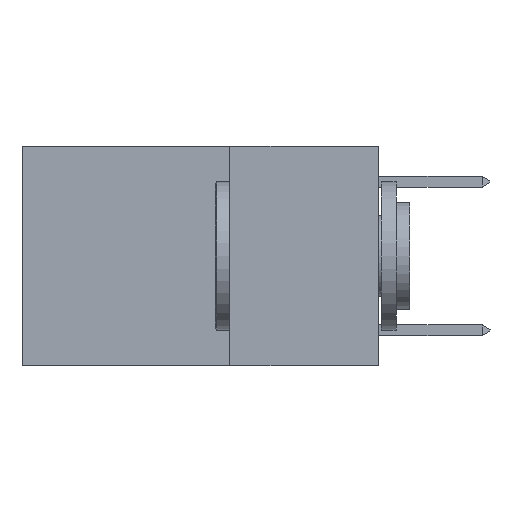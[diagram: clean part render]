
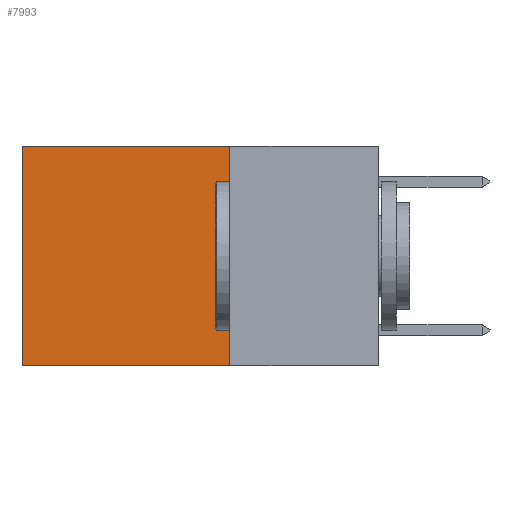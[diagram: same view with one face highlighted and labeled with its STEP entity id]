
A CAD part, left-side view. The second image highlights one B-rep face of the part: STEP entity #7993.
In plain terms, the highlighted planar face has unit normal (-1, 0, 0).
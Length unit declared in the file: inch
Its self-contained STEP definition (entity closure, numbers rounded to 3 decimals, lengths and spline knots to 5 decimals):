
#565 = CARTESIAN_POINT ( 'NONE',  ( 0.2625, 0.25, 0. ) ) ;
#1042 = DIRECTION ( 'NONE',  ( 0., 1., 0. ) ) ;
#1241 = CARTESIAN_POINT ( 'NONE',  ( 0.2625, 0.25, 0. ) ) ;
#1572 = VECTOR ( 'NONE', #13130, 39.37008 ) ;
#1951 = EDGE_CURVE ( 'NONE', #12552, #6987, #2225, .T. ) ;
#2107 = CARTESIAN_POINT ( 'NONE',  ( 0.2625, 0.6, 0. ) ) ;
#2225 = LINE ( 'NONE', #5620, #7541 ) ;
#2430 = PLANE ( 'NONE',  #9959 ) ;
#3626 = VERTEX_POINT ( 'NONE', #565 ) ;
#3913 = LINE ( 'NONE', #4499, #6541 ) ;
#4010 = DIRECTION ( 'NONE',  ( 0., 0., -1. ) ) ;
#4499 = CARTESIAN_POINT ( 'NONE',  ( 0.2625, 0.25, -0.37 ) ) ;
#4833 = EDGE_CURVE ( 'NONE', #3626, #13359, #7638, .T. ) ;
#5126 = CARTESIAN_POINT ( 'NONE',  ( 0.2625, 0.25, 0. ) ) ;
#5620 = CARTESIAN_POINT ( 'NONE',  ( 0.2625, 0.6, 0. ) ) ;
#5685 = ORIENTED_EDGE ( 'NONE', *, *, #6334, .F. ) ;
#5765 = CARTESIAN_POINT ( 'NONE',  ( 0.2625, 0.6, -0.37 ) ) ;
#6084 = LINE ( 'NONE', #5126, #14703 ) ;
#6334 = EDGE_CURVE ( 'NONE', #13359, #6987, #3913, .T. ) ;
#6541 = VECTOR ( 'NONE', #1042, 39.37008 ) ;
#6987 = VERTEX_POINT ( 'NONE', #5765 ) ;
#7541 = VECTOR ( 'NONE', #4010, 39.37008 ) ;
#7638 = LINE ( 'NONE', #12020, #1572 ) ;
#7993 = ADVANCED_FACE ( 'NONE', ( #12672 ), #2430, .F. ) ;
#8221 = EDGE_CURVE ( 'NONE', #3626, #12552, #6084, .T. ) ;
#9959 = AXIS2_PLACEMENT_3D ( 'NONE', #1241, #13712, #10430 ) ;
#10430 = DIRECTION ( 'NONE',  ( 0., 0., -1. ) ) ;
#11489 = ORIENTED_EDGE ( 'NONE', *, *, #4833, .F. ) ;
#11588 = EDGE_LOOP ( 'NONE', ( #12355, #5685, #11489, #13217 ) ) ;
#12020 = CARTESIAN_POINT ( 'NONE',  ( 0.2625, 0.25, 0. ) ) ;
#12355 = ORIENTED_EDGE ( 'NONE', *, *, #1951, .T. ) ;
#12552 = VERTEX_POINT ( 'NONE', #2107 ) ;
#12672 = FACE_OUTER_BOUND ( 'NONE', #11588, .T. ) ;
#13046 = DIRECTION ( 'NONE',  ( 0., 1., 0. ) ) ;
#13130 = DIRECTION ( 'NONE',  ( 0., 0., -1. ) ) ;
#13217 = ORIENTED_EDGE ( 'NONE', *, *, #8221, .T. ) ;
#13233 = CARTESIAN_POINT ( 'NONE',  ( 0.2625, 0.25, -0.37 ) ) ;
#13359 = VERTEX_POINT ( 'NONE', #13233 ) ;
#13712 = DIRECTION ( 'NONE',  ( 1., 0., 0. ) ) ;
#14703 = VECTOR ( 'NONE', #13046, 39.37008 ) ;
